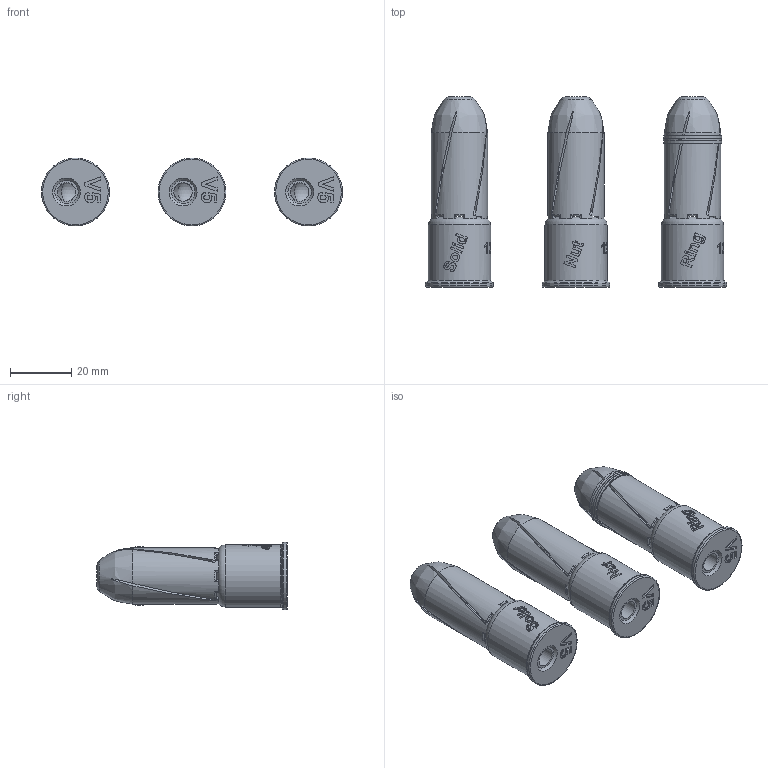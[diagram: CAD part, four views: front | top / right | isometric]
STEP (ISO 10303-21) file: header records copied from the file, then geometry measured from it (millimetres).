
FILE_DESCRIPTION(/* description */ (''),/* implementation_level */ '2;1');
FILE_NAME(/* name */ '12ga Blank Fired Slug.step',/* time_stamp */ '2022-03-12T15:59:32-05:00',/* author */ (''),/* organization */ (''),/* preprocessor_version */ 'ST-DEVELOPER v18.1',/* originating_system */ 'Autodesk Translation Framework v10.13.0.1454',/* authorisation */ '');
FILE_SCHEMA (('AUTOMOTIVE_DESIGN { 1 0 10303 214 3 1 1 }'));
Length unit declared in the file: inch
Products named in the file (1): 12ga Blank Slug
Bounding box: 98.42 x 62.23 x 22.23 mm (x, y, z)
Volume: 42324.5 mm3; surface area: 18906.1 mm2
Topology: 6 solids, 7 shells, 891 faces, 2604 edges, 1745 vertices
Faces by surface type: bspline 434, plane 322, cylinder 93, torus 27, cone 9, sphere 6
Full cylindrical faces by diameter (mm): 6.096 x3, 7.747 x1, 18.415 x3, 20.345 x3, 22.225 x3
Entity records: 39767 total; most frequent: CARTESIAN_POINT 18791, ORIENTED_EDGE 5202, DIRECTION 3031, EDGE_CURVE 2601, VERTEX_POINT 1745, B_SPLINE_CURVE_WITH_KNOTS 1035, LINE 1017, VECTOR 1017
